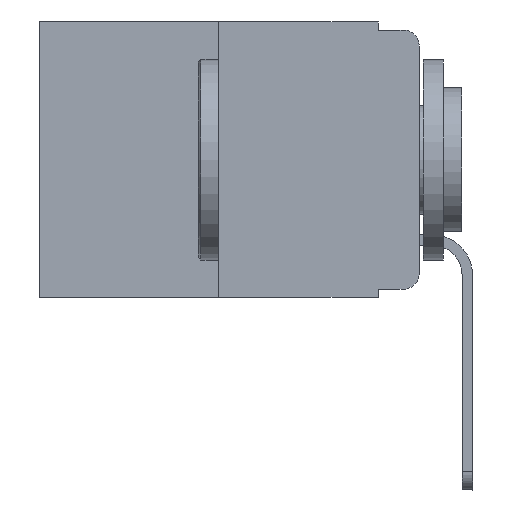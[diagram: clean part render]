
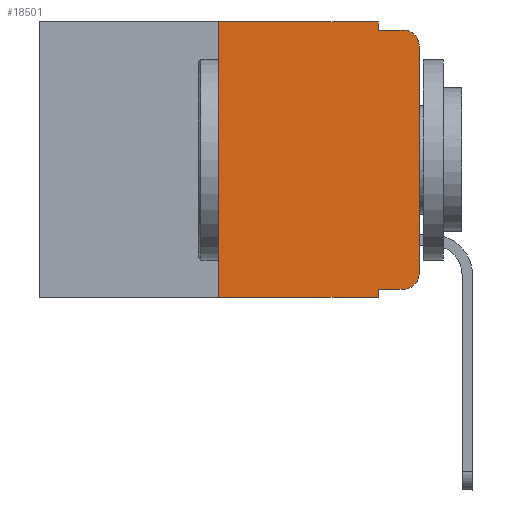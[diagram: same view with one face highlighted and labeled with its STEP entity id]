
A CAD part, left-side view. The second image highlights one B-rep face of the part: STEP entity #18501.
In plain terms, the highlighted planar face has unit normal (-1, 0, 0).
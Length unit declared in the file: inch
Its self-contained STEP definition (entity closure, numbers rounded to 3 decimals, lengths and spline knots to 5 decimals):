
#470 = VECTOR ( 'NONE', #2275, 39.37008 ) ;
#697 = VECTOR ( 'NONE', #11202, 39.37008 ) ;
#1051 = VERTEX_POINT ( 'NONE', #2733 ) ;
#1276 = AXIS2_PLACEMENT_3D ( 'NONE', #9820, #17690, #1851 ) ;
#1575 = DIRECTION ( 'NONE',  ( 0., 0., -1. ) ) ;
#1577 = CARTESIAN_POINT ( 'NONE',  ( 0., 0.051, -0.01 ) ) ;
#1764 = ORIENTED_EDGE ( 'NONE', *, *, #11230, .T. ) ;
#1851 = DIRECTION ( 'NONE',  ( 0., 0., -1. ) ) ;
#2275 = DIRECTION ( 'NONE',  ( 0., 0., 1. ) ) ;
#2368 = ORIENTED_EDGE ( 'NONE', *, *, #6343, .T. ) ;
#2559 = CARTESIAN_POINT ( 'NONE',  ( 0., 0.25, 0. ) ) ;
#2566 = ORIENTED_EDGE ( 'NONE', *, *, #10568, .T. ) ;
#2597 = CARTESIAN_POINT ( 'NONE',  ( 0., 0.02, -0.333 ) ) ;
#2606 = ORIENTED_EDGE ( 'NONE', *, *, #16383, .T. ) ;
#2640 = CIRCLE ( 'NONE', #1276, 0.02 ) ;
#2733 = CARTESIAN_POINT ( 'NONE',  ( 0., 0.051, -0.343 ) ) ;
#2770 = DIRECTION ( 'NONE',  ( 0., -1., 0. ) ) ;
#3084 = DIRECTION ( 'NONE',  ( -1., 0., 0. ) ) ;
#3191 = CARTESIAN_POINT ( 'NONE',  ( 0., 0.02, -0.03 ) ) ;
#4245 = LINE ( 'NONE', #12412, #5741 ) ;
#4448 = DIRECTION ( 'NONE',  ( 0., -1., 0. ) ) ;
#4565 = VECTOR ( 'NONE', #2770, 39.37008 ) ;
#4997 = VECTOR ( 'NONE', #14601, 39.37008 ) ;
#5146 = CARTESIAN_POINT ( 'NONE',  ( 0., 0.473, 0. ) ) ;
#5229 = EDGE_LOOP ( 'NONE', ( #2368, #1764, #19032, #19885, #6354, #11509, #2566, #12391, #2606, #15821 ) ) ;
#5674 = EDGE_CURVE ( 'NONE', #20145, #19111, #17520, .T. ) ;
#5741 = VECTOR ( 'NONE', #4448, 39.37008 ) ;
#5819 = CARTESIAN_POINT ( 'NONE',  ( 0., 0.051, 0. ) ) ;
#6193 = VECTOR ( 'NONE', #16523, 39.37008 ) ;
#6248 = CARTESIAN_POINT ( 'NONE',  ( 0., 0.051, -0.333 ) ) ;
#6308 = LINE ( 'NONE', #16286, #697 ) ;
#6343 = EDGE_CURVE ( 'NONE', #14901, #11314, #6639, .T. ) ;
#6354 = ORIENTED_EDGE ( 'NONE', *, *, #14469, .F. ) ;
#6363 = CARTESIAN_POINT ( 'NONE',  ( 0., 0., -0.03 ) ) ;
#6639 = LINE ( 'NONE', #7382, #470 ) ;
#7367 = PLANE ( 'NONE',  #11538 ) ;
#7382 = CARTESIAN_POINT ( 'NONE',  ( 0., 0., 0. ) ) ;
#7683 = CARTESIAN_POINT ( 'NONE',  ( 0., 0.25, -0.343 ) ) ;
#8109 = CARTESIAN_POINT ( 'NONE',  ( 0., 0., -0.313 ) ) ;
#8708 = LINE ( 'NONE', #5819, #16399 ) ;
#9141 = EDGE_CURVE ( 'NONE', #11556, #20145, #6308, .T. ) ;
#9820 = CARTESIAN_POINT ( 'NONE',  ( 0., 0.02, -0.313 ) ) ;
#9903 = EDGE_CURVE ( 'NONE', #11955, #20604, #13719, .T. ) ;
#9961 = LINE ( 'NONE', #11535, #6193 ) ;
#10128 = CARTESIAN_POINT ( 'NONE',  ( 0., 0.25, 0. ) ) ;
#10448 = DIRECTION ( 'NONE',  ( 0., 0., -1. ) ) ;
#10515 = DIRECTION ( 'NONE',  ( 0., 0., 1. ) ) ;
#10568 = EDGE_CURVE ( 'NONE', #11955, #1051, #9961, .T. ) ;
#11202 = DIRECTION ( 'NONE',  ( 0., 0., -1. ) ) ;
#11230 = EDGE_CURVE ( 'NONE', #11314, #19111, #16730, .T. ) ;
#11314 = VERTEX_POINT ( 'NONE', #6363 ) ;
#11503 = EDGE_CURVE ( 'NONE', #17826, #1051, #8708, .T. ) ;
#11509 = ORIENTED_EDGE ( 'NONE', *, *, #9903, .F. ) ;
#11535 = CARTESIAN_POINT ( 'NONE',  ( 0., 0.473, -0.343 ) ) ;
#11538 = AXIS2_PLACEMENT_3D ( 'NONE', #13850, #13755, #10448 ) ;
#11556 = VERTEX_POINT ( 'NONE', #20092 ) ;
#11955 = VERTEX_POINT ( 'NONE', #7683 ) ;
#12391 = ORIENTED_EDGE ( 'NONE', *, *, #11503, .F. ) ;
#12412 = CARTESIAN_POINT ( 'NONE',  ( 0., 0.051, -0.333 ) ) ;
#13065 = EDGE_CURVE ( 'NONE', #19705, #14901, #2640, .T. ) ;
#13242 = CARTESIAN_POINT ( 'NONE',  ( 0., 0.02, -0.01 ) ) ;
#13719 = LINE ( 'NONE', #2559, #20112 ) ;
#13755 = DIRECTION ( 'NONE',  ( 1., 0., 0. ) ) ;
#13850 = CARTESIAN_POINT ( 'NONE',  ( 0., 0.473, 0. ) ) ;
#13960 = FACE_OUTER_BOUND ( 'NONE', #5229, .T. ) ;
#14469 = EDGE_CURVE ( 'NONE', #20604, #11556, #19415, .T. ) ;
#14601 = DIRECTION ( 'NONE',  ( 0., -1., 0. ) ) ;
#14901 = VERTEX_POINT ( 'NONE', #8109 ) ;
#15032 = AXIS2_PLACEMENT_3D ( 'NONE', #3191, #3084, #1575 ) ;
#15821 = ORIENTED_EDGE ( 'NONE', *, *, #13065, .T. ) ;
#16286 = CARTESIAN_POINT ( 'NONE',  ( 0., 0.051, 0. ) ) ;
#16383 = EDGE_CURVE ( 'NONE', #17826, #19705, #4245, .T. ) ;
#16399 = VECTOR ( 'NONE', #18910, 39.37008 ) ;
#16523 = DIRECTION ( 'NONE',  ( 0., -1., 0. ) ) ;
#16730 = CIRCLE ( 'NONE', #15032, 0.02 ) ;
#17520 = LINE ( 'NONE', #20733, #4565 ) ;
#17690 = DIRECTION ( 'NONE',  ( -1., 0., 0. ) ) ;
#17826 = VERTEX_POINT ( 'NONE', #6248 ) ;
#18501 = ADVANCED_FACE ( 'NONE', ( #13960 ), #7367, .F. ) ;
#18910 = DIRECTION ( 'NONE',  ( 0., 0., -1. ) ) ;
#19032 = ORIENTED_EDGE ( 'NONE', *, *, #5674, .F. ) ;
#19111 = VERTEX_POINT ( 'NONE', #13242 ) ;
#19415 = LINE ( 'NONE', #5146, #4997 ) ;
#19705 = VERTEX_POINT ( 'NONE', #2597 ) ;
#19885 = ORIENTED_EDGE ( 'NONE', *, *, #9141, .F. ) ;
#20092 = CARTESIAN_POINT ( 'NONE',  ( 0., 0.051, 0. ) ) ;
#20112 = VECTOR ( 'NONE', #10515, 39.37008 ) ;
#20145 = VERTEX_POINT ( 'NONE', #1577 ) ;
#20604 = VERTEX_POINT ( 'NONE', #10128 ) ;
#20733 = CARTESIAN_POINT ( 'NONE',  ( 0., 0.051, -0.01 ) ) ;
